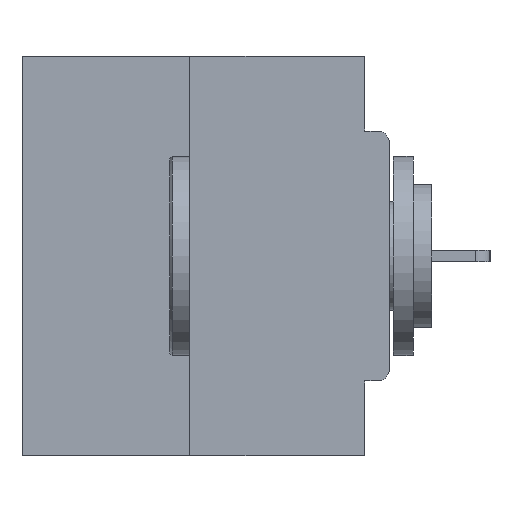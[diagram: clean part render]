
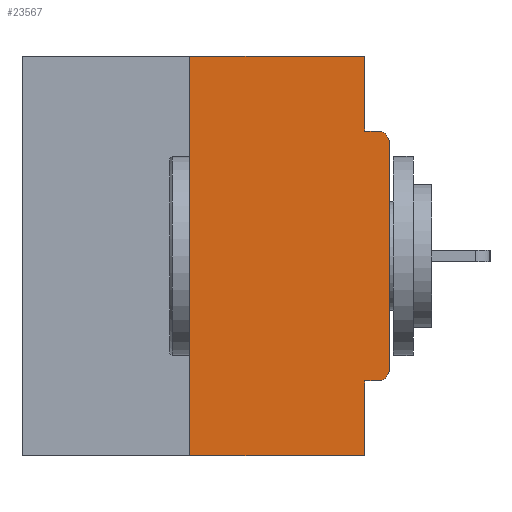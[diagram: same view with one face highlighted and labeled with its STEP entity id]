
A CAD part, left-side view. The second image highlights one B-rep face of the part: STEP entity #23567.
In plain terms, the highlighted planar face has unit normal (-1, 0, 0).
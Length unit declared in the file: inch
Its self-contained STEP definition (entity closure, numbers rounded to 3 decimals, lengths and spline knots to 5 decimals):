
#524 = VECTOR ( 'NONE', #10649, 39.37008 ) ;
#1475 = VECTOR ( 'NONE', #7835, 39.37008 ) ;
#2131 = VECTOR ( 'NONE', #7540, 39.37008 ) ;
#2209 = LINE ( 'NONE', #12544, #2131 ) ;
#2438 = EDGE_CURVE ( 'NONE', #5536, #21146, #5643, .T. ) ;
#2440 = CARTESIAN_POINT ( 'NONE',  ( 0., 0.25, 0. ) ) ;
#2937 = VERTEX_POINT ( 'NONE', #12128 ) ;
#2958 = CARTESIAN_POINT ( 'NONE',  ( 0., 0., -0.0935 ) ) ;
#3131 = VERTEX_POINT ( 'NONE', #10609 ) ;
#3343 = CARTESIAN_POINT ( 'NONE',  ( 0., 0.46, 0. ) ) ;
#3690 = LINE ( 'NONE', #10883, #13388 ) ;
#3783 = ORIENTED_EDGE ( 'NONE', *, *, #20774, .T. ) ;
#3820 = AXIS2_PLACEMENT_3D ( 'NONE', #28514, #23684, #24007 ) ;
#4105 = CARTESIAN_POINT ( 'NONE',  ( 0., 0.015, -0.4065 ) ) ;
#4448 = EDGE_LOOP ( 'NONE', ( #5152, #20656, #18033, #10045, #30107, #8029, #3783, #32346, #31225, #29971 ) ) ;
#4730 = DIRECTION ( 'NONE',  ( 0., 0., -1. ) ) ;
#5152 = ORIENTED_EDGE ( 'NONE', *, *, #8302, .F. ) ;
#5536 = VERTEX_POINT ( 'NONE', #15675 ) ;
#5643 = LINE ( 'NONE', #15814, #524 ) ;
#5829 = LINE ( 'NONE', #28525, #1475 ) ;
#7540 = DIRECTION ( 'NONE',  ( 0., 0., -1. ) ) ;
#7835 = DIRECTION ( 'NONE',  ( 0., 0., 1. ) ) ;
#8029 = ORIENTED_EDGE ( 'NONE', *, *, #15902, .T. ) ;
#8187 = DIRECTION ( 'NONE',  ( 0., -1., 0. ) ) ;
#8302 = EDGE_CURVE ( 'NONE', #19891, #5536, #28680, .T. ) ;
#8558 = VERTEX_POINT ( 'NONE', #9332 ) ;
#9332 = CARTESIAN_POINT ( 'NONE',  ( 0., 0.015, -0.0935 ) ) ;
#9727 = DIRECTION ( 'NONE',  ( 0., 0., -1. ) ) ;
#10045 = ORIENTED_EDGE ( 'NONE', *, *, #31685, .F. ) ;
#10065 = FACE_OUTER_BOUND ( 'NONE', #4448, .T. ) ;
#10463 = LINE ( 'NONE', #2958, #18741 ) ;
#10609 = CARTESIAN_POINT ( 'NONE',  ( 0., 0.25, -0.5 ) ) ;
#10649 = DIRECTION ( 'NONE',  ( 0., 0., -1. ) ) ;
#10660 = AXIS2_PLACEMENT_3D ( 'NONE', #12571, #15232, #4730 ) ;
#10699 = EDGE_CURVE ( 'NONE', #3131, #19891, #25797, .T. ) ;
#10883 = CARTESIAN_POINT ( 'NONE',  ( 0., 0.46, -0.5 ) ) ;
#11114 = DIRECTION ( 'NONE',  ( 0., -1., 0. ) ) ;
#12128 = CARTESIAN_POINT ( 'NONE',  ( 0., 0., -0.3915 ) ) ;
#12338 = CIRCLE ( 'NONE', #3820, 0.015 ) ;
#12544 = CARTESIAN_POINT ( 'NONE',  ( 0., 0.031, -0.5 ) ) ;
#12571 = CARTESIAN_POINT ( 'NONE',  ( 0., 0.46, 0. ) ) ;
#13388 = VECTOR ( 'NONE', #18380, 39.37008 ) ;
#14710 = CARTESIAN_POINT ( 'NONE',  ( 0., 0., -0.1085 ) ) ;
#15232 = DIRECTION ( 'NONE',  ( 1., 0., 0. ) ) ;
#15432 = EDGE_CURVE ( 'NONE', #3131, #21114, #3690, .T. ) ;
#15675 = CARTESIAN_POINT ( 'NONE',  ( 0., 0.031, 0. ) ) ;
#15814 = CARTESIAN_POINT ( 'NONE',  ( 0., 0.031, 0. ) ) ;
#15902 = EDGE_CURVE ( 'NONE', #17763, #2937, #12338, .T. ) ;
#16314 = EDGE_CURVE ( 'NONE', #21146, #8558, #10463, .T. ) ;
#17763 = VERTEX_POINT ( 'NONE', #4105 ) ;
#17816 = CARTESIAN_POINT ( 'NONE',  ( 0., 0.031, -0.5 ) ) ;
#17997 = VECTOR ( 'NONE', #28113, 39.37008 ) ;
#18033 = ORIENTED_EDGE ( 'NONE', *, *, #15432, .T. ) ;
#18380 = DIRECTION ( 'NONE',  ( 0., -1., 0. ) ) ;
#18741 = VECTOR ( 'NONE', #11114, 39.37008 ) ;
#18861 = CARTESIAN_POINT ( 'NONE',  ( 0., 0., -0.4065 ) ) ;
#19891 = VERTEX_POINT ( 'NONE', #21259 ) ;
#20091 = PLANE ( 'NONE',  #10660 ) ;
#20656 = ORIENTED_EDGE ( 'NONE', *, *, #10699, .F. ) ;
#20774 = EDGE_CURVE ( 'NONE', #2937, #27401, #5829, .T. ) ;
#21114 = VERTEX_POINT ( 'NONE', #17816 ) ;
#21146 = VERTEX_POINT ( 'NONE', #32486 ) ;
#21259 = CARTESIAN_POINT ( 'NONE',  ( 0., 0.25, 0. ) ) ;
#21547 = DIRECTION ( 'NONE',  ( 0., 1., 0. ) ) ;
#23567 = ADVANCED_FACE ( 'NONE', ( #10065 ), #20091, .F. ) ;
#23684 = DIRECTION ( 'NONE',  ( -1., 0., 0. ) ) ;
#24007 = DIRECTION ( 'NONE',  ( 0., 0., -1. ) ) ;
#25797 = LINE ( 'NONE', #2440, #17997 ) ;
#26230 = LINE ( 'NONE', #18861, #26675 ) ;
#26627 = AXIS2_PLACEMENT_3D ( 'NONE', #30065, #27256, #9727 ) ;
#26675 = VECTOR ( 'NONE', #21547, 39.37008 ) ;
#27147 = CIRCLE ( 'NONE', #26627, 0.015 ) ;
#27256 = DIRECTION ( 'NONE',  ( -1., 0., 0. ) ) ;
#27401 = VERTEX_POINT ( 'NONE', #14710 ) ;
#28113 = DIRECTION ( 'NONE',  ( 0., 0., 1. ) ) ;
#28478 = VERTEX_POINT ( 'NONE', #32081 ) ;
#28514 = CARTESIAN_POINT ( 'NONE',  ( 0., 0.015, -0.3915 ) ) ;
#28525 = CARTESIAN_POINT ( 'NONE',  ( 0., 0., 0. ) ) ;
#28680 = LINE ( 'NONE', #3343, #30378 ) ;
#29755 = EDGE_CURVE ( 'NONE', #27401, #8558, #27147, .T. ) ;
#29971 = ORIENTED_EDGE ( 'NONE', *, *, #2438, .F. ) ;
#30065 = CARTESIAN_POINT ( 'NONE',  ( 0., 0.015, -0.1085 ) ) ;
#30107 = ORIENTED_EDGE ( 'NONE', *, *, #30832, .F. ) ;
#30378 = VECTOR ( 'NONE', #8187, 39.37008 ) ;
#30832 = EDGE_CURVE ( 'NONE', #17763, #28478, #26230, .T. ) ;
#31225 = ORIENTED_EDGE ( 'NONE', *, *, #16314, .F. ) ;
#31685 = EDGE_CURVE ( 'NONE', #28478, #21114, #2209, .T. ) ;
#32081 = CARTESIAN_POINT ( 'NONE',  ( 0., 0.031, -0.4065 ) ) ;
#32346 = ORIENTED_EDGE ( 'NONE', *, *, #29755, .T. ) ;
#32486 = CARTESIAN_POINT ( 'NONE',  ( 0., 0.031, -0.0935 ) ) ;
